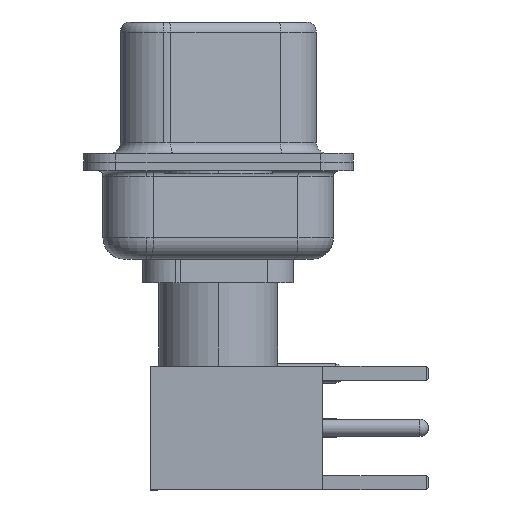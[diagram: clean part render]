
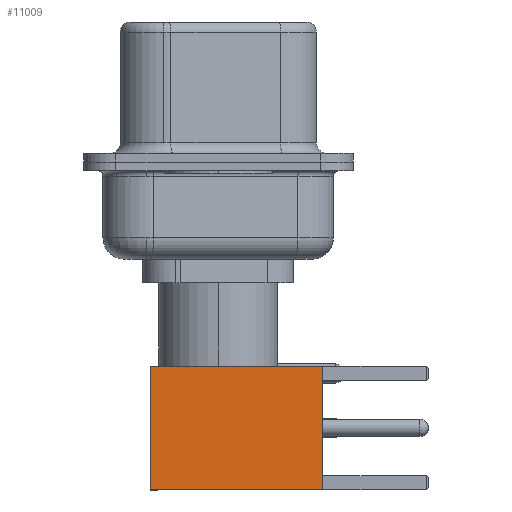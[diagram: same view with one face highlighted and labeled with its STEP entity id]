
A CAD part, left-side view. The second image highlights one B-rep face of the part: STEP entity #11009.
In plain terms, the highlighted face is planar.
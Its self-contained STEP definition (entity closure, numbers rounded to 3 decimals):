
#256 = VERTEX_POINT ( 'NONE', #13768 ) ;
#546 = DIRECTION ( 'NONE',  ( 0., 0., -1. ) ) ;
#1430 = ORIENTED_EDGE ( 'NONE', *, *, #14603, .F. ) ;
#1648 = CARTESIAN_POINT ( 'NONE',  ( 2.875, 2.875, 0. ) ) ;
#1949 = VECTOR ( 'NONE', #8611, 1000. ) ;
#2233 = VERTEX_POINT ( 'NONE', #2672 ) ;
#2392 = EDGE_CURVE ( 'NONE', #21014, #256, #4306, .T. ) ;
#2672 = CARTESIAN_POINT ( 'NONE',  ( -2.875, 2.875, 8. ) ) ;
#4306 = LINE ( 'NONE', #8327, #17301 ) ;
#4662 = AXIS2_PLACEMENT_3D ( 'NONE', #1648, #18969, #12377 ) ;
#4964 = ORIENTED_EDGE ( 'NONE', *, *, #2392, .T. ) ;
#5712 = VECTOR ( 'NONE', #10773, 1000. ) ;
#8327 = CARTESIAN_POINT ( 'NONE',  ( 0., 2.875, 0. ) ) ;
#8468 = CARTESIAN_POINT ( 'NONE',  ( 2.875, 2.875, 8. ) ) ;
#8611 = DIRECTION ( 'NONE',  ( 0., 0., -1. ) ) ;
#10211 = VERTEX_POINT ( 'NONE', #8468 ) ;
#10773 = DIRECTION ( 'NONE',  ( -1., 0., 0. ) ) ;
#11009 = ADVANCED_FACE ( 'NONE', ( #12247 ), #14315, .T. ) ;
#12247 = FACE_OUTER_BOUND ( 'NONE', #18805, .T. ) ;
#12377 = DIRECTION ( 'NONE',  ( 0., 0., 1. ) ) ;
#12827 = CARTESIAN_POINT ( 'NONE',  ( 0., 2.875, 8. ) ) ;
#13768 = CARTESIAN_POINT ( 'NONE',  ( -2.875, 2.875, 0. ) ) ;
#14315 = PLANE ( 'NONE',  #4662 ) ;
#14603 = EDGE_CURVE ( 'NONE', #10211, #2233, #14910, .T. ) ;
#14609 = ORIENTED_EDGE ( 'NONE', *, *, #24898, .F. ) ;
#14863 = CARTESIAN_POINT ( 'NONE',  ( 2.875, 2.875, 0. ) ) ;
#14910 = LINE ( 'NONE', #12827, #5712 ) ;
#16834 = VECTOR ( 'NONE', #546, 1000. ) ;
#16857 = LINE ( 'NONE', #21113, #1949 ) ;
#17301 = VECTOR ( 'NONE', #26892, 1000. ) ;
#18805 = EDGE_LOOP ( 'NONE', ( #23304, #4964, #14609, #1430 ) ) ;
#18969 = DIRECTION ( 'NONE',  ( 0., 1., 0. ) ) ;
#19312 = EDGE_CURVE ( 'NONE', #10211, #21014, #25344, .T. ) ;
#21014 = VERTEX_POINT ( 'NONE', #14863 ) ;
#21113 = CARTESIAN_POINT ( 'NONE',  ( -2.875, 2.875, 0. ) ) ;
#23134 = CARTESIAN_POINT ( 'NONE',  ( 2.875, 2.875, 0. ) ) ;
#23304 = ORIENTED_EDGE ( 'NONE', *, *, #19312, .T. ) ;
#24898 = EDGE_CURVE ( 'NONE', #2233, #256, #16857, .T. ) ;
#25344 = LINE ( 'NONE', #23134, #16834 ) ;
#26892 = DIRECTION ( 'NONE',  ( -1., 0., 0. ) ) ;
